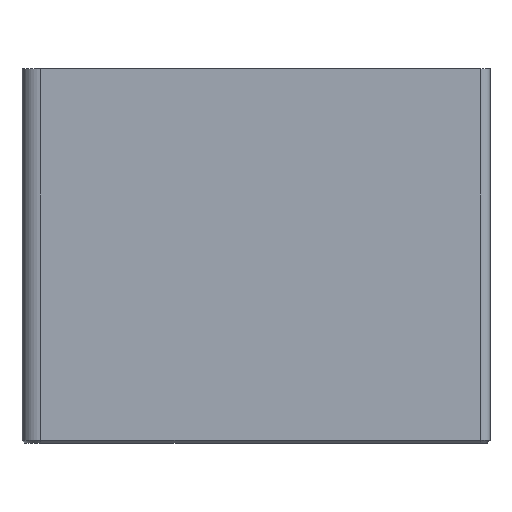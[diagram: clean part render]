
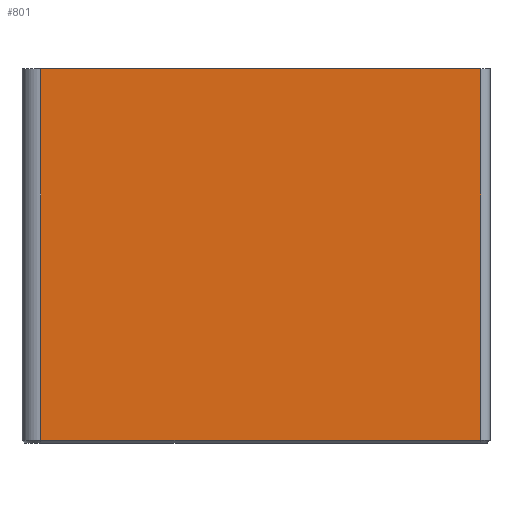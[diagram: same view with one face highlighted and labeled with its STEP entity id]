
A CAD part, front view. The second image highlights one B-rep face of the part: STEP entity #801.
In plain terms, the highlighted planar face has unit normal (0, -1, 0).
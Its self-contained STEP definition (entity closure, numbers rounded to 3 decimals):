
#58=PLANE('',#873);
#81=FACE_OUTER_BOUND('',#131,.T.);
#131=EDGE_LOOP('',(#577,#578,#579,#580));
#228=LINE('',#1251,#294);
#233=LINE('',#1264,#299);
#234=LINE('',#1266,#300);
#235=LINE('',#1267,#301);
#294=VECTOR('',#990,10.);
#299=VECTOR('',#1005,10.);
#300=VECTOR('',#1006,10.);
#301=VECTOR('',#1007,10.);
#360=VERTEX_POINT('',#1243);
#362=VERTEX_POINT('',#1249);
#365=VERTEX_POINT('',#1263);
#366=VERTEX_POINT('',#1265);
#440=EDGE_CURVE('',#362,#360,#228,.T.);
#447=EDGE_CURVE('',#365,#362,#233,.T.);
#448=EDGE_CURVE('',#366,#365,#234,.T.);
#449=EDGE_CURVE('',#360,#366,#235,.T.);
#577=ORIENTED_EDGE('',*,*,#440,.F.);
#578=ORIENTED_EDGE('',*,*,#447,.F.);
#579=ORIENTED_EDGE('',*,*,#448,.F.);
#580=ORIENTED_EDGE('',*,*,#449,.F.);
#801=ADVANCED_FACE('',(#81),#58,.T.);
#873=AXIS2_PLACEMENT_3D('',#1262,#1003,#1004);
#990=DIRECTION('',(-1.,0.,0.));
#1003=DIRECTION('center_axis',(0.,-1.,0.));
#1004=DIRECTION('ref_axis',(1.,0.,0.));
#1005=DIRECTION('',(0.,0.,-1.));
#1006=DIRECTION('',(1.,0.,0.));
#1007=DIRECTION('',(0.,0.,1.));
#1243=CARTESIAN_POINT('',(-2.,-4.,0.3));
#1249=CARTESIAN_POINT('',(45.,-4.,0.3));
#1251=CARTESIAN_POINT('',(8.5,-4.,0.3));
#1262=CARTESIAN_POINT('Origin',(-4.,-4.,0.));
#1263=CARTESIAN_POINT('',(45.,-4.,40.));
#1264=CARTESIAN_POINT('',(45.,-4.,0.));
#1265=CARTESIAN_POINT('',(-2.,-4.,40.));
#1266=CARTESIAN_POINT('',(-4.,-4.,40.));
#1267=CARTESIAN_POINT('',(-2.,-4.,0.));
